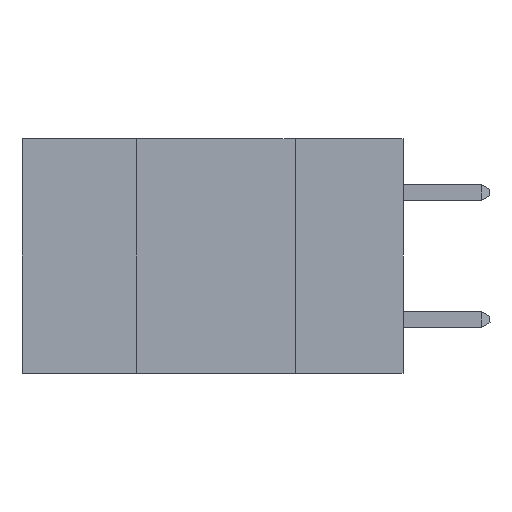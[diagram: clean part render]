
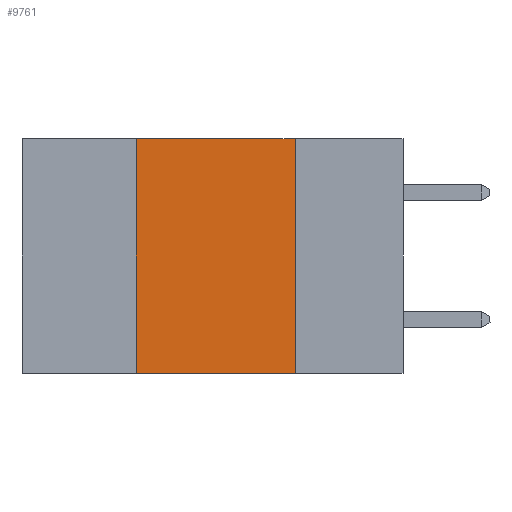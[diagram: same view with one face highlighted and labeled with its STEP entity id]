
A CAD part, left-side view. The second image highlights one B-rep face of the part: STEP entity #9761.
In plain terms, the highlighted planar face has unit normal (-1, 0, 0).
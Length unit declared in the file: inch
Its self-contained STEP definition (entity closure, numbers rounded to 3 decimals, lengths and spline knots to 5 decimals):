
#232 = CARTESIAN_POINT ( 'NONE',  ( 0., 0.42, 0. ) ) ;
#1466 = EDGE_CURVE ( 'NONE', #7200, #5948, #3750, .T. ) ;
#1697 = DIRECTION ( 'NONE',  ( 0., 0., -1. ) ) ;
#2106 = PLANE ( 'NONE',  #13003 ) ;
#3274 = EDGE_LOOP ( 'NONE', ( #4116, #7990, #16622, #13245 ) ) ;
#3683 = CARTESIAN_POINT ( 'NONE',  ( 0., 0.42, 0. ) ) ;
#3750 = LINE ( 'NONE', #17516, #15369 ) ;
#4116 = ORIENTED_EDGE ( 'NONE', *, *, #11855, .F. ) ;
#5948 = VERTEX_POINT ( 'NONE', #12649 ) ;
#6451 = DIRECTION ( 'NONE',  ( 0., 0., -1. ) ) ;
#7200 = VERTEX_POINT ( 'NONE', #3683 ) ;
#7990 = ORIENTED_EDGE ( 'NONE', *, *, #1466, .F. ) ;
#9761 = ADVANCED_FACE ( 'NONE', ( #17167 ), #2106, .F. ) ;
#10115 = DIRECTION ( 'NONE',  ( 0., -1., 0. ) ) ;
#10150 = EDGE_CURVE ( 'NONE', #18431, #7200, #14677, .T. ) ;
#11855 = EDGE_CURVE ( 'NONE', #5948, #16185, #18456, .T. ) ;
#11893 = DIRECTION ( 'NONE',  ( 0., 0., 1. ) ) ;
#12356 = EDGE_CURVE ( 'NONE', #18431, #16185, #17958, .T. ) ;
#12602 = DIRECTION ( 'NONE',  ( 0., -1., 0. ) ) ;
#12649 = CARTESIAN_POINT ( 'NONE',  ( 0., 0.17, 0. ) ) ;
#13003 = AXIS2_PLACEMENT_3D ( 'NONE', #13723, #15185, #6451 ) ;
#13245 = ORIENTED_EDGE ( 'NONE', *, *, #12356, .T. ) ;
#13723 = CARTESIAN_POINT ( 'NONE',  ( 0., 0.6, 0. ) ) ;
#14149 = VECTOR ( 'NONE', #10115, 39.37008 ) ;
#14608 = VECTOR ( 'NONE', #1697, 39.37008 ) ;
#14677 = LINE ( 'NONE', #232, #18060 ) ;
#15185 = DIRECTION ( 'NONE',  ( 1., 0., 0. ) ) ;
#15369 = VECTOR ( 'NONE', #12602, 39.37008 ) ;
#15854 = CARTESIAN_POINT ( 'NONE',  ( 0., 0.6, -0.37 ) ) ;
#16113 = CARTESIAN_POINT ( 'NONE',  ( 0., 0.42, -0.37 ) ) ;
#16180 = CARTESIAN_POINT ( 'NONE',  ( 0., 0.17, 0. ) ) ;
#16185 = VERTEX_POINT ( 'NONE', #16785 ) ;
#16622 = ORIENTED_EDGE ( 'NONE', *, *, #10150, .F. ) ;
#16785 = CARTESIAN_POINT ( 'NONE',  ( 0., 0.17, -0.37 ) ) ;
#17167 = FACE_OUTER_BOUND ( 'NONE', #3274, .T. ) ;
#17516 = CARTESIAN_POINT ( 'NONE',  ( 0., 0.6, 0. ) ) ;
#17958 = LINE ( 'NONE', #15854, #14149 ) ;
#18060 = VECTOR ( 'NONE', #11893, 39.37008 ) ;
#18431 = VERTEX_POINT ( 'NONE', #16113 ) ;
#18456 = LINE ( 'NONE', #16180, #14608 ) ;
